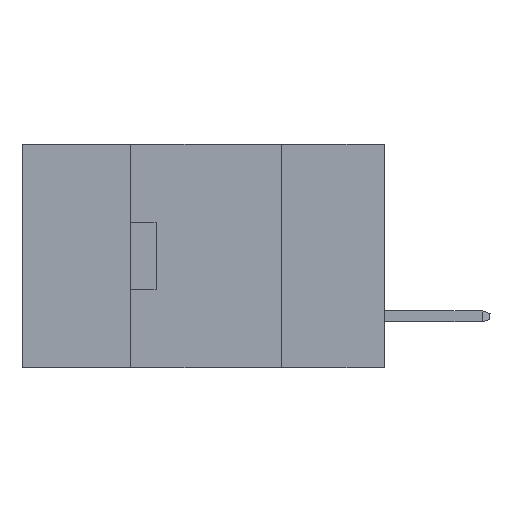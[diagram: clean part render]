
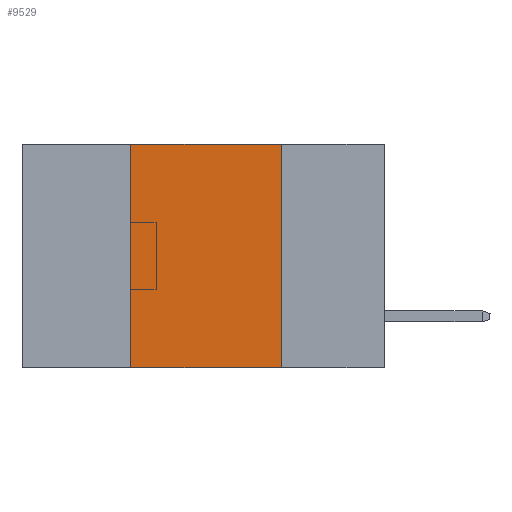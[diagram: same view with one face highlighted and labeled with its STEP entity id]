
A CAD part, left-side view. The second image highlights one B-rep face of the part: STEP entity #9529.
In plain terms, the highlighted planar face has unit normal (-1, 0, 0).
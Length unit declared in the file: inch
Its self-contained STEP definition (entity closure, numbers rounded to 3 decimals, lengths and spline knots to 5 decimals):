
#377 = DIRECTION ( 'NONE',  ( 0., -1., 0. ) ) ;
#1411 = CARTESIAN_POINT ( 'NONE',  ( 0., 0.42, -0.37 ) ) ;
#1419 = LINE ( 'NONE', #20242, #1602 ) ;
#1602 = VECTOR ( 'NONE', #7526, 39.37008 ) ;
#2448 = CARTESIAN_POINT ( 'NONE',  ( 0., 0.6, -0.37 ) ) ;
#3983 = CARTESIAN_POINT ( 'NONE',  ( 0., 0.6, 0. ) ) ;
#5667 = FACE_OUTER_BOUND ( 'NONE', #13007, .T. ) ;
#6446 = EDGE_CURVE ( 'NONE', #8923, #20232, #1419, .T. ) ;
#7471 = CARTESIAN_POINT ( 'NONE',  ( 0., 0.17, -0.37 ) ) ;
#7526 = DIRECTION ( 'NONE',  ( 0., -1., 0. ) ) ;
#8923 = VERTEX_POINT ( 'NONE', #19804 ) ;
#9010 = EDGE_CURVE ( 'NONE', #18984, #8923, #20506, .T. ) ;
#9529 = ADVANCED_FACE ( 'NONE', ( #5667 ), #11948, .F. ) ;
#9562 = DIRECTION ( 'NONE',  ( 0., 0., -1. ) ) ;
#9865 = DIRECTION ( 'NONE',  ( 1., 0., 0. ) ) ;
#10131 = DIRECTION ( 'NONE',  ( 0., 0., -1. ) ) ;
#11938 = LINE ( 'NONE', #7471, #17277 ) ;
#11948 = PLANE ( 'NONE',  #24379 ) ;
#12866 = ORIENTED_EDGE ( 'NONE', *, *, #15138, .F. ) ;
#13007 = EDGE_LOOP ( 'NONE', ( #12866, #21969, #24863, #25287 ) ) ;
#14994 = LINE ( 'NONE', #2448, #17437 ) ;
#15138 = EDGE_CURVE ( 'NONE', #20232, #22964, #11938, .T. ) ;
#15336 = VECTOR ( 'NONE', #25119, 39.37008 ) ;
#15426 = CARTESIAN_POINT ( 'NONE',  ( 0., 0.42, -0.37 ) ) ;
#16295 = CARTESIAN_POINT ( 'NONE',  ( 0., 0.17, -0.37 ) ) ;
#17277 = VECTOR ( 'NONE', #9562, 39.37008 ) ;
#17437 = VECTOR ( 'NONE', #377, 39.37008 ) ;
#18984 = VERTEX_POINT ( 'NONE', #15426 ) ;
#19804 = CARTESIAN_POINT ( 'NONE',  ( 0., 0.42, 0. ) ) ;
#20232 = VERTEX_POINT ( 'NONE', #25621 ) ;
#20242 = CARTESIAN_POINT ( 'NONE',  ( 0., 0.6, 0. ) ) ;
#20506 = LINE ( 'NONE', #1411, #15336 ) ;
#21969 = ORIENTED_EDGE ( 'NONE', *, *, #6446, .F. ) ;
#22964 = VERTEX_POINT ( 'NONE', #16295 ) ;
#23101 = EDGE_CURVE ( 'NONE', #18984, #22964, #14994, .T. ) ;
#24379 = AXIS2_PLACEMENT_3D ( 'NONE', #3983, #9865, #10131 ) ;
#24863 = ORIENTED_EDGE ( 'NONE', *, *, #9010, .F. ) ;
#25119 = DIRECTION ( 'NONE',  ( 0., 0., 1. ) ) ;
#25287 = ORIENTED_EDGE ( 'NONE', *, *, #23101, .T. ) ;
#25621 = CARTESIAN_POINT ( 'NONE',  ( 0., 0.17, 0. ) ) ;
